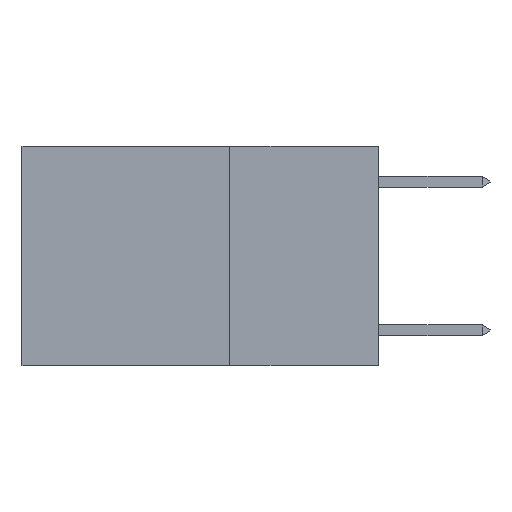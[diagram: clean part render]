
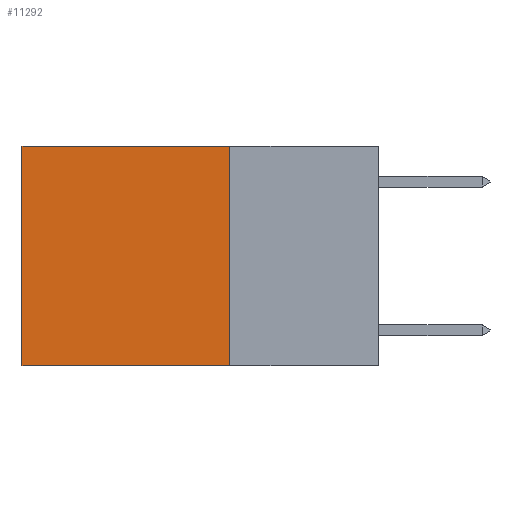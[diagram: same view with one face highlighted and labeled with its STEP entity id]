
A CAD part, left-side view. The second image highlights one B-rep face of the part: STEP entity #11292.
In plain terms, the highlighted planar face has unit normal (-1, 0, 0).
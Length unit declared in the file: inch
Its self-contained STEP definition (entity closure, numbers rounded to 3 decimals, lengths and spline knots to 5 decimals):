
#190 = EDGE_LOOP ( 'NONE', ( #7033, #1910, #11606, #4568 ) ) ;
#455 = LINE ( 'NONE', #6544, #9778 ) ;
#749 = VECTOR ( 'NONE', #3591, 39.37008 ) ;
#839 = LINE ( 'NONE', #4432, #9207 ) ;
#1726 = FACE_OUTER_BOUND ( 'NONE', #190, .T. ) ;
#1910 = ORIENTED_EDGE ( 'NONE', *, *, #6492, .F. ) ;
#3192 = CARTESIAN_POINT ( 'NONE',  ( 0.2625, 0.25, 0. ) ) ;
#3298 = CARTESIAN_POINT ( 'NONE',  ( 0.2625, 0.25, 0. ) ) ;
#3591 = DIRECTION ( 'NONE',  ( 0., 0., -1. ) ) ;
#4033 = DIRECTION ( 'NONE',  ( 0., 0., -1. ) ) ;
#4432 = CARTESIAN_POINT ( 'NONE',  ( 0.2625, 0.6, 0. ) ) ;
#4442 = CARTESIAN_POINT ( 'NONE',  ( 0.2625, 0.25, 0. ) ) ;
#4568 = ORIENTED_EDGE ( 'NONE', *, *, #5096, .T. ) ;
#4613 = CARTESIAN_POINT ( 'NONE',  ( 0.2625, 0.6, 0. ) ) ;
#4656 = EDGE_CURVE ( 'NONE', #10123, #6953, #839, .T. ) ;
#4867 = CARTESIAN_POINT ( 'NONE',  ( 0.2625, 0.6, -0.37 ) ) ;
#4883 = DIRECTION ( 'NONE',  ( 0., 1., 0. ) ) ;
#5096 = EDGE_CURVE ( 'NONE', #11138, #10123, #7251, .T. ) ;
#5273 = PLANE ( 'NONE',  #10964 ) ;
#6096 = CARTESIAN_POINT ( 'NONE',  ( 0.2625, 0.25, 0. ) ) ;
#6492 = EDGE_CURVE ( 'NONE', #10414, #6953, #455, .T. ) ;
#6544 = CARTESIAN_POINT ( 'NONE',  ( 0.2625, 0.25, -0.37 ) ) ;
#6953 = VERTEX_POINT ( 'NONE', #4867 ) ;
#7033 = ORIENTED_EDGE ( 'NONE', *, *, #4656, .T. ) ;
#7251 = LINE ( 'NONE', #3192, #8332 ) ;
#7623 = DIRECTION ( 'NONE',  ( 0., 1., 0. ) ) ;
#7974 = LINE ( 'NONE', #6096, #749 ) ;
#8145 = EDGE_CURVE ( 'NONE', #11138, #10414, #7974, .T. ) ;
#8332 = VECTOR ( 'NONE', #4883, 39.37008 ) ;
#8906 = CARTESIAN_POINT ( 'NONE',  ( 0.2625, 0.25, -0.37 ) ) ;
#8919 = DIRECTION ( 'NONE',  ( 1., 0., 0. ) ) ;
#9207 = VECTOR ( 'NONE', #4033, 39.37008 ) ;
#9778 = VECTOR ( 'NONE', #7623, 39.37008 ) ;
#9854 = DIRECTION ( 'NONE',  ( 0., 0., -1. ) ) ;
#10123 = VERTEX_POINT ( 'NONE', #4613 ) ;
#10414 = VERTEX_POINT ( 'NONE', #8906 ) ;
#10964 = AXIS2_PLACEMENT_3D ( 'NONE', #4442, #8919, #9854 ) ;
#11138 = VERTEX_POINT ( 'NONE', #3298 ) ;
#11292 = ADVANCED_FACE ( 'NONE', ( #1726 ), #5273, .F. ) ;
#11606 = ORIENTED_EDGE ( 'NONE', *, *, #8145, .F. ) ;
